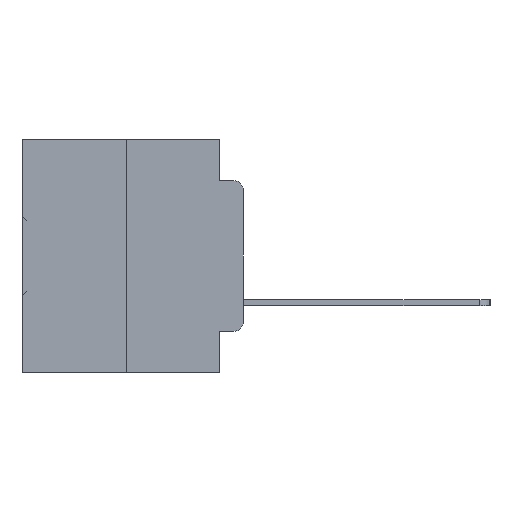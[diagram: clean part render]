
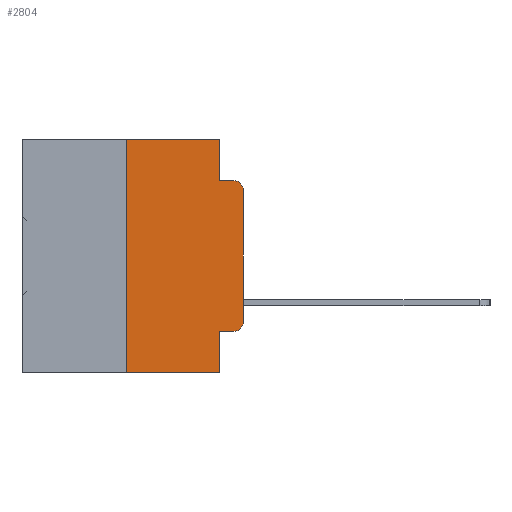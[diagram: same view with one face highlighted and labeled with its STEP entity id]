
A CAD part, left-side view. The second image highlights one B-rep face of the part: STEP entity #2804.
In plain terms, the highlighted planar face has unit normal (-1, 0, 0).
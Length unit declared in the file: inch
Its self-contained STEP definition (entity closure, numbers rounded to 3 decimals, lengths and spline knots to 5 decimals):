
#970 = ORIENTED_EDGE ( 'NONE', *, *, #7053, .F. ) ;
#2309 = ORIENTED_EDGE ( 'NONE', *, *, #27996, .T. ) ;
#2312 = CARTESIAN_POINT ( 'NONE',  ( 0., 0.051, -0.0885 ) ) ;
#2718 = CARTESIAN_POINT ( 'NONE',  ( 0., 0.473, -0.5 ) ) ;
#2727 = VERTEX_POINT ( 'NONE', #17328 ) ;
#2728 = VECTOR ( 'NONE', #14249, 39.37008 ) ;
#2731 = ORIENTED_EDGE ( 'NONE', *, *, #5166, .F. ) ;
#2804 = ADVANCED_FACE ( 'NONE', ( #8069 ), #15827, .F. ) ;
#2999 = CARTESIAN_POINT ( 'NONE',  ( 0., 0.051, 0. ) ) ;
#4074 = VERTEX_POINT ( 'NONE', #28922 ) ;
#4086 = VECTOR ( 'NONE', #29690, 39.37008 ) ;
#4105 = VERTEX_POINT ( 'NONE', #7170 ) ;
#4129 = VECTOR ( 'NONE', #29919, 39.37008 ) ;
#5042 = VERTEX_POINT ( 'NONE', #30373 ) ;
#5166 = EDGE_CURVE ( 'NONE', #32987, #4105, #15219, .T. ) ;
#5794 = CARTESIAN_POINT ( 'NONE',  ( 0., 0.051, -0.4115 ) ) ;
#6563 = VECTOR ( 'NONE', #8910, 39.37008 ) ;
#6607 = CARTESIAN_POINT ( 'NONE',  ( 0., 0.02, -0.3915 ) ) ;
#7053 = EDGE_CURVE ( 'NONE', #4105, #32033, #33407, .T. ) ;
#7052 = CARTESIAN_POINT ( 'NONE',  ( 0., 0.02, -0.4115 ) ) ;
#7170 = CARTESIAN_POINT ( 'NONE',  ( 0., 0.051, -0.0885 ) ) ;
#7726 = CARTESIAN_POINT ( 'NONE',  ( 0., 0., 0. ) ) ;
#8069 = FACE_OUTER_BOUND ( 'NONE', #23079, .T. ) ;
#8162 = LINE ( 'NONE', #10093, #35605 ) ;
#8460 = DIRECTION ( 'NONE',  ( -1., 0., 0. ) ) ;
#8748 = AXIS2_PLACEMENT_3D ( 'NONE', #6607, #25877, #9420 ) ;
#8910 = DIRECTION ( 'NONE',  ( 0., 0., 1. ) ) ;
#8917 = EDGE_CURVE ( 'NONE', #5042, #32033, #32400, .T. ) ;
#8921 = DIRECTION ( 'NONE',  ( 0., 0., -1. ) ) ;
#9420 = DIRECTION ( 'NONE',  ( 0., 0., -1. ) ) ;
#10093 = CARTESIAN_POINT ( 'NONE',  ( 0., 0.051, -0.4115 ) ) ;
#10208 = LINE ( 'NONE', #2999, #2728 ) ;
#10831 = CARTESIAN_POINT ( 'NONE',  ( 0., 0.02, -0.0885 ) ) ;
#11788 = LINE ( 'NONE', #31146, #24677 ) ;
#12339 = AXIS2_PLACEMENT_3D ( 'NONE', #19436, #20909, #20799 ) ;
#12648 = EDGE_CURVE ( 'NONE', #4074, #5042, #18931, .T. ) ;
#12802 = ORIENTED_EDGE ( 'NONE', *, *, #25116, .F. ) ;
#13251 = VERTEX_POINT ( 'NONE', #26798 ) ;
#14249 = DIRECTION ( 'NONE',  ( 0., 0., -1. ) ) ;
#15219 = LINE ( 'NONE', #30854, #28872 ) ;
#15827 = PLANE ( 'NONE',  #12339 ) ;
#17328 = CARTESIAN_POINT ( 'NONE',  ( 0., 0.25, -0.5 ) ) ;
#17601 = ORIENTED_EDGE ( 'NONE', *, *, #35305, .F. ) ;
#18931 = LINE ( 'NONE', #7726, #4086 ) ;
#19436 = CARTESIAN_POINT ( 'NONE',  ( 0., 0.473, 0. ) ) ;
#20799 = DIRECTION ( 'NONE',  ( 0., 0., -1. ) ) ;
#20909 = DIRECTION ( 'NONE',  ( 1., 0., 0. ) ) ;
#21901 = ORIENTED_EDGE ( 'NONE', *, *, #33480, .F. ) ;
#22004 = LINE ( 'NONE', #2718, #34704 ) ;
#22188 = DIRECTION ( 'NONE',  ( 0., -1., 0. ) ) ;
#23070 = CARTESIAN_POINT ( 'NONE',  ( 0., 0.051, 0. ) ) ;
#23079 = EDGE_LOOP ( 'NONE', ( #30739, #31184, #970, #2731, #12802, #17601, #28217, #21901, #23592, #2309 ) ) ;
#23592 = ORIENTED_EDGE ( 'NONE', *, *, #31641, .T. ) ;
#24677 = VECTOR ( 'NONE', #33887, 39.37008 ) ;
#24948 = CARTESIAN_POINT ( 'NONE',  ( 0., 0.02, -0.1085 ) ) ;
#24967 = VERTEX_POINT ( 'NONE', #5794 ) ;
#25116 = EDGE_CURVE ( 'NONE', #13251, #32987, #11788, .T. ) ;
#25393 = CARTESIAN_POINT ( 'NONE',  ( 0., 0.25, 0. ) ) ;
#25696 = CARTESIAN_POINT ( 'NONE',  ( 0., 0.051, -0.5 ) ) ;
#25877 = DIRECTION ( 'NONE',  ( -1., 0., 0. ) ) ;
#26131 = CIRCLE ( 'NONE', #8748, 0.02 ) ;
#26798 = CARTESIAN_POINT ( 'NONE',  ( 0., 0.25, 0. ) ) ;
#26822 = VERTEX_POINT ( 'NONE', #7052 ) ;
#27615 = AXIS2_PLACEMENT_3D ( 'NONE', #24948, #8460, #27668 ) ;
#27634 = LINE ( 'NONE', #25393, #6563 ) ;
#27668 = DIRECTION ( 'NONE',  ( 0., 0., -1. ) ) ;
#27996 = EDGE_CURVE ( 'NONE', #26822, #4074, #26131, .T. ) ;
#28217 = ORIENTED_EDGE ( 'NONE', *, *, #32104, .T. ) ;
#28872 = VECTOR ( 'NONE', #8921, 39.37008 ) ;
#28922 = CARTESIAN_POINT ( 'NONE',  ( 0., 0., -0.3915 ) ) ;
#29690 = DIRECTION ( 'NONE',  ( 0., 0., 1. ) ) ;
#29919 = DIRECTION ( 'NONE',  ( 0., -1., 0. ) ) ;
#30373 = CARTESIAN_POINT ( 'NONE',  ( 0., 0., -0.1085 ) ) ;
#30739 = ORIENTED_EDGE ( 'NONE', *, *, #12648, .T. ) ;
#30854 = CARTESIAN_POINT ( 'NONE',  ( 0., 0.051, 0. ) ) ;
#31146 = CARTESIAN_POINT ( 'NONE',  ( 0., 0.473, 0. ) ) ;
#31184 = ORIENTED_EDGE ( 'NONE', *, *, #8917, .T. ) ;
#31641 = EDGE_CURVE ( 'NONE', #24967, #26822, #8162, .T. ) ;
#31965 = DIRECTION ( 'NONE',  ( 0., -1., 0. ) ) ;
#32033 = VERTEX_POINT ( 'NONE', #10831 ) ;
#32104 = EDGE_CURVE ( 'NONE', #2727, #34095, #22004, .T. ) ;
#32400 = CIRCLE ( 'NONE', #27615, 0.02 ) ;
#32987 = VERTEX_POINT ( 'NONE', #23070 ) ;
#33407 = LINE ( 'NONE', #2312, #4129 ) ;
#33480 = EDGE_CURVE ( 'NONE', #24967, #34095, #10208, .T. ) ;
#33887 = DIRECTION ( 'NONE',  ( 0., -1., 0. ) ) ;
#34095 = VERTEX_POINT ( 'NONE', #25696 ) ;
#34704 = VECTOR ( 'NONE', #22188, 39.37008 ) ;
#35305 = EDGE_CURVE ( 'NONE', #2727, #13251, #27634, .T. ) ;
#35605 = VECTOR ( 'NONE', #31965, 39.37008 ) ;
